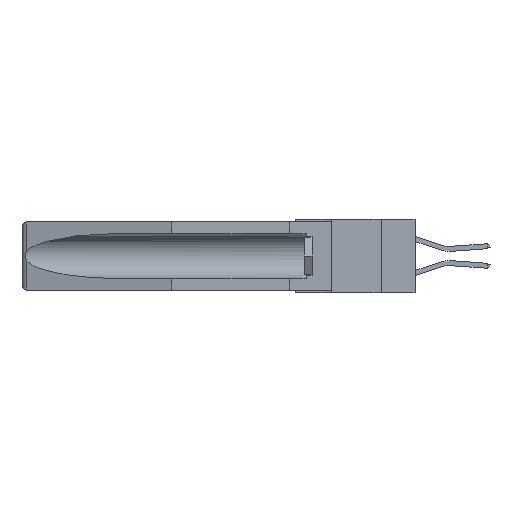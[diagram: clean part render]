
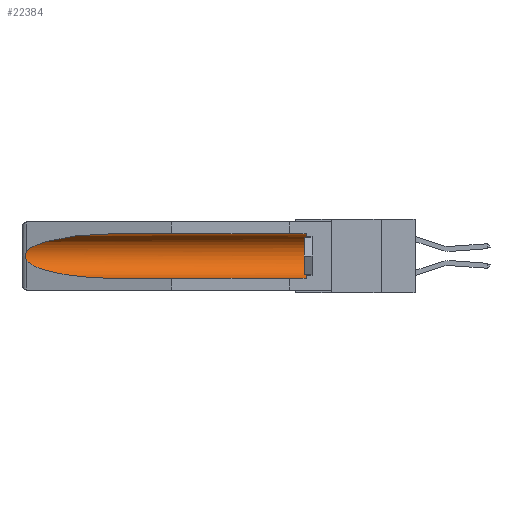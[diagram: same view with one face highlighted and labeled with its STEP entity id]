
A CAD part, left-side view. The second image highlights one B-rep face of the part: STEP entity #22384.
In plain terms, the highlighted cylindrical face has radius 2.857 mm (diameter 5.715 mm), a partial arc.
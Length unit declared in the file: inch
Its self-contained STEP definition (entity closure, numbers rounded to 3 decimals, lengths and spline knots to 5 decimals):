
#613 = CARTESIAN_POINT ( 'NONE',  ( 0.155, 0.126, -0.284 ) ) ;
#760 = CARTESIAN_POINT ( 'NONE',  ( 0.21114, 1.30732, -0.059 ) ) ;
#1449 = ORIENTED_EDGE ( 'NONE', *, *, #15913, .T. ) ;
#1559 = ORIENTED_EDGE ( 'NONE', *, *, #4866, .T. ) ;
#1655 = CARTESIAN_POINT ( 'NONE',  ( 0.2675, 1.53308, -0.16763 ) ) ;
#2012 = CARTESIAN_POINT ( 'NONE',  ( 0.21114, 1.30732, -0.284 ) ) ;
#2503 =( BOUNDED_CURVE ( )  B_SPLINE_CURVE ( 3, ( #20206, #5601, #2012, #22144 ),
 .UNSPECIFIED., .F., .F. ) 
 B_SPLINE_CURVE_WITH_KNOTS ( ( 4, 4 ),
 ( 0.1948, 1.5708 ),
 .UNSPECIFIED. ) 
 CURVE ( )  GEOMETRIC_REPRESENTATION_ITEM ( )  RATIONAL_B_SPLINE_CURVE ( ( 1., 0.848, 0.848, 1. ) ) 
 REPRESENTATION_ITEM ( '' )  );
#2886 = CARTESIAN_POINT ( 'NONE',  ( 0.26537, 1.52718, -0.14972 ) ) ;
#3175 = CARTESIAN_POINT ( 'NONE',  ( 0.2673, 1.53269, -0.17917 ) ) ;
#3253 = CARTESIAN_POINT ( 'NONE',  ( 0.2673, 1.5327, -0.16383 ) ) ;
#3402 = CARTESIAN_POINT ( 'NONE',  ( 0.26537, 1.52718, -0.19328 ) ) ;
#4021 = EDGE_LOOP ( 'NONE', ( #9995, #1449, #6868, #19234, #1559, #23242 ) ) ;
#4866 = EDGE_CURVE ( 'NONE', #5203, #6927, #14490, .T. ) ;
#5176 = EDGE_CURVE ( 'NONE', #6927, #6121, #5636, .T. ) ;
#5203 = VERTEX_POINT ( 'NONE', #613 ) ;
#5471 = CARTESIAN_POINT ( 'NONE',  ( 0.155, -0.30754, -0.284 ) ) ;
#5555 = DIRECTION ( 'NONE',  ( 0., 1., 0. ) ) ;
#5601 = CARTESIAN_POINT ( 'NONE',  ( 0.25451, 1.48313, -0.24835 ) ) ;
#5636 = LINE ( 'NONE', #11475, #15628 ) ;
#6013 = DIRECTION ( 'NONE',  ( 0., 1., 0. ) ) ;
#6089 = EDGE_CURVE ( 'NONE', #5203, #17839, #10584, .T. ) ;
#6121 = VERTEX_POINT ( 'NONE', #10823 ) ;
#6325 = EDGE_CURVE ( 'NONE', #6121, #18233, #16267, .T. ) ;
#6665 = CARTESIAN_POINT ( 'NONE',  ( 0.26537, 1.52718, -0.19328 ) ) ;
#6868 = ORIENTED_EDGE ( 'NONE', *, *, #8865, .T. ) ;
#6927 = VERTEX_POINT ( 'NONE', #16004 ) ;
#7936 = CARTESIAN_POINT ( 'NONE',  ( 0.155, 1.07973, -0.059 ) ) ;
#8865 = EDGE_CURVE ( 'NONE', #19468, #17839, #2503, .T. ) ;
#9685 = AXIS2_PLACEMENT_3D ( 'NONE', #15915, #17828, #21486 ) ;
#9995 = ORIENTED_EDGE ( 'NONE', *, *, #6325, .T. ) ;
#10457 = CARTESIAN_POINT ( 'NONE',  ( 0.26654, 1.53092, -0.15636 ) ) ;
#10537 = CARTESIAN_POINT ( 'NONE',  ( 0.26655, 1.53094, -0.18657 ) ) ;
#10584 = LINE ( 'NONE', #5471, #15730 ) ;
#10823 = CARTESIAN_POINT ( 'NONE',  ( 0.155, 1.07973, -0.059 ) ) ;
#10966 = CARTESIAN_POINT ( 'NONE',  ( 0.155, 0.126, -0.1715 ) ) ;
#11052 = DIRECTION ( 'NONE',  ( 0., -1., 0. ) ) ;
#11475 = CARTESIAN_POINT ( 'NONE',  ( 0.155, -0.30754, -0.059 ) ) ;
#11969 = CARTESIAN_POINT ( 'NONE',  ( 0.155, 1.07973, -0.284 ) ) ;
#12039 = AXIS2_PLACEMENT_3D ( 'NONE', #10966, #11052, #12872 ) ;
#12872 = DIRECTION ( 'NONE',  ( 0., 0., 1. ) ) ;
#14490 = CIRCLE ( 'NONE', #12039, 0.1125 ) ;
#14831 = B_SPLINE_CURVE_WITH_KNOTS ( 'NONE', 3,
 ( #19856, #23314, #10457, #3253, #1655, #23544, #3175, #10537, #17875, #3402 ),
 .UNSPECIFIED., .F., .F.,
 ( 4, 2, 2, 2, 4 ),
 ( 0., 0.00029, 0.00058, 0.00087, 0.00117 ),
 .UNSPECIFIED. ) ;
#15628 = VECTOR ( 'NONE', #6013, 39.37008 ) ;
#15730 = VECTOR ( 'NONE', #5555, 39.37008 ) ;
#15913 = EDGE_CURVE ( 'NONE', #18233, #19468, #14831, .T. ) ;
#15915 = CARTESIAN_POINT ( 'NONE',  ( 0.155, -0.30754, -0.1715 ) ) ;
#16004 = CARTESIAN_POINT ( 'NONE',  ( 0.155, 0.126, -0.059 ) ) ;
#16267 =( BOUNDED_CURVE ( )  B_SPLINE_CURVE ( 3, ( #7936, #760, #22854, #2886 ),
 .UNSPECIFIED., .F., .F. ) 
 B_SPLINE_CURVE_WITH_KNOTS ( ( 4, 4 ),
 ( 4.71239, 6.08839 ),
 .UNSPECIFIED. ) 
 CURVE ( )  GEOMETRIC_REPRESENTATION_ITEM ( )  RATIONAL_B_SPLINE_CURVE ( ( 1., 0.848, 0.848, 1. ) ) 
 REPRESENTATION_ITEM ( '' )  );
#17828 = DIRECTION ( 'NONE',  ( 0., 1., 0. ) ) ;
#17839 = VERTEX_POINT ( 'NONE', #11969 ) ;
#17875 = CARTESIAN_POINT ( 'NONE',  ( 0.26597, 1.5296, -0.19026 ) ) ;
#18233 = VERTEX_POINT ( 'NONE', #22930 ) ;
#19234 = ORIENTED_EDGE ( 'NONE', *, *, #6089, .F. ) ;
#19319 = CYLINDRICAL_SURFACE ( 'NONE', #9685, 0.1125 ) ;
#19468 = VERTEX_POINT ( 'NONE', #6665 ) ;
#19600 = FACE_OUTER_BOUND ( 'NONE', #4021, .T. ) ;
#19856 = CARTESIAN_POINT ( 'NONE',  ( 0.26537, 1.52718, -0.14972 ) ) ;
#20206 = CARTESIAN_POINT ( 'NONE',  ( 0.26537, 1.52718, -0.19328 ) ) ;
#21486 = DIRECTION ( 'NONE',  ( 0., 0., 1. ) ) ;
#22144 = CARTESIAN_POINT ( 'NONE',  ( 0.155, 1.07973, -0.284 ) ) ;
#22384 = ADVANCED_FACE ( 'NONE', ( #19600 ), #19319, .F. ) ;
#22854 = CARTESIAN_POINT ( 'NONE',  ( 0.25451, 1.48313, -0.09465 ) ) ;
#22930 = CARTESIAN_POINT ( 'NONE',  ( 0.26537, 1.52718, -0.14972 ) ) ;
#23242 = ORIENTED_EDGE ( 'NONE', *, *, #5176, .T. ) ;
#23314 = CARTESIAN_POINT ( 'NONE',  ( 0.26597, 1.52961, -0.15275 ) ) ;
#23544 = CARTESIAN_POINT ( 'NONE',  ( 0.2675, 1.53308, -0.17534 ) ) ;
